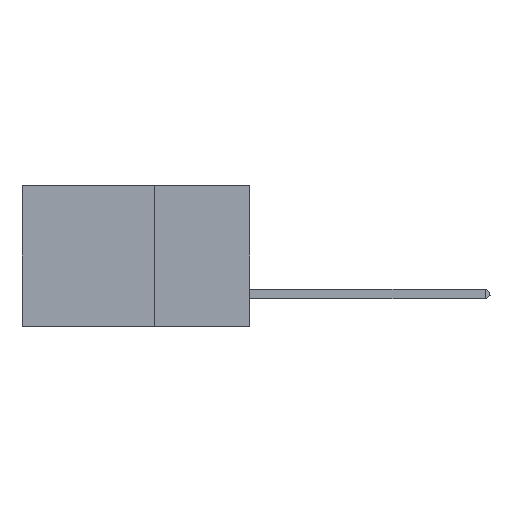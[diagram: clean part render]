
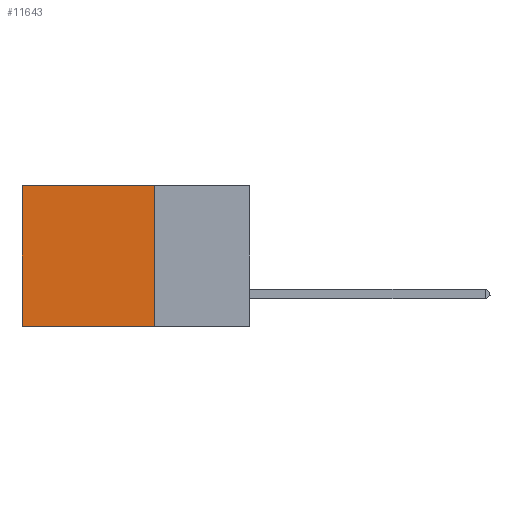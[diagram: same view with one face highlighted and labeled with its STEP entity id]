
A CAD part, left-side view. The second image highlights one B-rep face of the part: STEP entity #11643.
In plain terms, the highlighted planar face has unit normal (-1, 0, 0).
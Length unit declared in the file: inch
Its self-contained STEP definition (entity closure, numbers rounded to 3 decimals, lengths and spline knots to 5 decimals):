
#29 = ORIENTED_EDGE ( 'NONE', *, *, #2729, .T. ) ;
#549 = FACE_OUTER_BOUND ( 'NONE', #34822, .T. ) ;
#2496 = DIRECTION ( 'NONE',  ( 0., 0., -1. ) ) ;
#2729 = EDGE_CURVE ( 'NONE', #30142, #31254, #17612, .T. ) ;
#3633 = EDGE_CURVE ( 'NONE', #31254, #24658, #11880, .T. ) ;
#3734 = CARTESIAN_POINT ( 'NONE',  ( 0.2875, 0.6, 0. ) ) ;
#4304 = CARTESIAN_POINT ( 'NONE',  ( 0.2875, 0.25, 0. ) ) ;
#4868 = DIRECTION ( 'NONE',  ( 0., 0., -1. ) ) ;
#8025 = DIRECTION ( 'NONE',  ( 0., 0., -1. ) ) ;
#8211 = CARTESIAN_POINT ( 'NONE',  ( 0.2875, 0.25, -0.37 ) ) ;
#11643 = ADVANCED_FACE ( 'NONE', ( #549 ), #18747, .F. ) ;
#11880 = LINE ( 'NONE', #24355, #34355 ) ;
#13800 = VERTEX_POINT ( 'NONE', #8211 ) ;
#16320 = VECTOR ( 'NONE', #28363, 39.37008 ) ;
#17477 = CARTESIAN_POINT ( 'NONE',  ( 0.2875, 0.25, -0.37 ) ) ;
#17607 = DIRECTION ( 'NONE',  ( 0., 1., 0. ) ) ;
#17612 = LINE ( 'NONE', #28491, #16320 ) ;
#17643 = EDGE_CURVE ( 'NONE', #30142, #13800, #24515, .T. ) ;
#17797 = AXIS2_PLACEMENT_3D ( 'NONE', #32221, #23912, #4868 ) ;
#18021 = ORIENTED_EDGE ( 'NONE', *, *, #31300, .F. ) ;
#18747 = PLANE ( 'NONE',  #17797 ) ;
#21522 = VECTOR ( 'NONE', #17607, 39.37008 ) ;
#23912 = DIRECTION ( 'NONE',  ( 1., 0., 0. ) ) ;
#24355 = CARTESIAN_POINT ( 'NONE',  ( 0.2875, 0.6, 0. ) ) ;
#24515 = LINE ( 'NONE', #30092, #30940 ) ;
#24658 = VERTEX_POINT ( 'NONE', #32325 ) ;
#28363 = DIRECTION ( 'NONE',  ( 0., 1., 0. ) ) ;
#28491 = CARTESIAN_POINT ( 'NONE',  ( 0.2875, 0.25, 0. ) ) ;
#30092 = CARTESIAN_POINT ( 'NONE',  ( 0.2875, 0.25, 0. ) ) ;
#30141 = LINE ( 'NONE', #17477, #21522 ) ;
#30142 = VERTEX_POINT ( 'NONE', #4304 ) ;
#30940 = VECTOR ( 'NONE', #8025, 39.37008 ) ;
#31200 = ORIENTED_EDGE ( 'NONE', *, *, #17643, .F. ) ;
#31254 = VERTEX_POINT ( 'NONE', #3734 ) ;
#31300 = EDGE_CURVE ( 'NONE', #13800, #24658, #30141, .T. ) ;
#32221 = CARTESIAN_POINT ( 'NONE',  ( 0.2875, 0.25, 0. ) ) ;
#32325 = CARTESIAN_POINT ( 'NONE',  ( 0.2875, 0.6, -0.37 ) ) ;
#34355 = VECTOR ( 'NONE', #2496, 39.37008 ) ;
#34822 = EDGE_LOOP ( 'NONE', ( #34875, #18021, #31200, #29 ) ) ;
#34875 = ORIENTED_EDGE ( 'NONE', *, *, #3633, .T. ) ;
